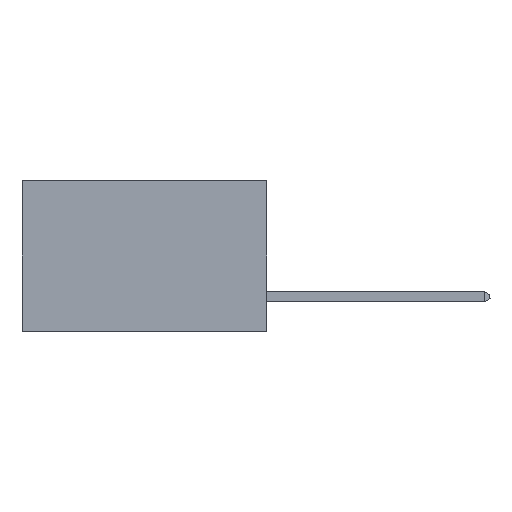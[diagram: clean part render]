
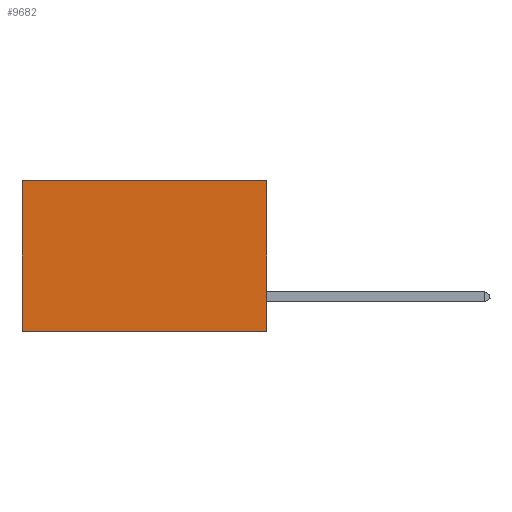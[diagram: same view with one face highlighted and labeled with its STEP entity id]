
A CAD part, left-side view. The second image highlights one B-rep face of the part: STEP entity #9682.
In plain terms, the highlighted planar face has unit normal (-1, 0, 0).
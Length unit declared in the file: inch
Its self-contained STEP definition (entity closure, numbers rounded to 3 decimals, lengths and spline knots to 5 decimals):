
#956 = CARTESIAN_POINT ( 'NONE',  ( 0.2875, 0., -0.37 ) ) ;
#1392 = EDGE_CURVE ( 'NONE', #4689, #6636, #9210, .T. ) ;
#2105 = CARTESIAN_POINT ( 'NONE',  ( 0.2875, 0., 0. ) ) ;
#2436 = CARTESIAN_POINT ( 'NONE',  ( 0.2875, 0.6, 0. ) ) ;
#4689 = VERTEX_POINT ( 'NONE', #9300 ) ;
#6636 = VERTEX_POINT ( 'NONE', #956 ) ;
#9111 = ORIENTED_EDGE ( 'NONE', *, *, #23193, .T. ) ;
#9210 = LINE ( 'NONE', #2105, #10890 ) ;
#9248 = CARTESIAN_POINT ( 'NONE',  ( 0.2875, 0.6, -0.37 ) ) ;
#9300 = CARTESIAN_POINT ( 'NONE',  ( 0.2875, 0., 0. ) ) ;
#9354 = LINE ( 'NONE', #16980, #9716 ) ;
#9682 = ADVANCED_FACE ( 'NONE', ( #26703 ), #21024, .F. ) ;
#9716 = VECTOR ( 'NONE', #25395, 39.37008 ) ;
#10189 = DIRECTION ( 'NONE',  ( 0., 0., -1. ) ) ;
#10890 = VECTOR ( 'NONE', #22115, 39.37008 ) ;
#11216 = DIRECTION ( 'NONE',  ( 0., 0., -1. ) ) ;
#11293 = LINE ( 'NONE', #2436, #22869 ) ;
#15219 = EDGE_CURVE ( 'NONE', #6636, #17281, #9354, .T. ) ;
#16893 = CARTESIAN_POINT ( 'NONE',  ( 0.2875, 0., 0. ) ) ;
#16980 = CARTESIAN_POINT ( 'NONE',  ( 0.2875, 0., -0.37 ) ) ;
#17281 = VERTEX_POINT ( 'NONE', #9248 ) ;
#17890 = EDGE_LOOP ( 'NONE', ( #9111, #19348, #21341, #23915 ) ) ;
#18639 = LINE ( 'NONE', #23963, #24464 ) ;
#18724 = DIRECTION ( 'NONE',  ( 1., 0., 0. ) ) ;
#19348 = ORIENTED_EDGE ( 'NONE', *, *, #15219, .F. ) ;
#21024 = PLANE ( 'NONE',  #23832 ) ;
#21341 = ORIENTED_EDGE ( 'NONE', *, *, #1392, .F. ) ;
#21384 = EDGE_CURVE ( 'NONE', #4689, #22201, #18639, .T. ) ;
#22115 = DIRECTION ( 'NONE',  ( 0., 0., -1. ) ) ;
#22201 = VERTEX_POINT ( 'NONE', #22796 ) ;
#22796 = CARTESIAN_POINT ( 'NONE',  ( 0.2875, 0.6, 0. ) ) ;
#22869 = VECTOR ( 'NONE', #11216, 39.37008 ) ;
#23193 = EDGE_CURVE ( 'NONE', #22201, #17281, #11293, .T. ) ;
#23832 = AXIS2_PLACEMENT_3D ( 'NONE', #16893, #18724, #10189 ) ;
#23915 = ORIENTED_EDGE ( 'NONE', *, *, #21384, .T. ) ;
#23963 = CARTESIAN_POINT ( 'NONE',  ( 0.2875, 0., 0. ) ) ;
#24464 = VECTOR ( 'NONE', #26182, 39.37008 ) ;
#25395 = DIRECTION ( 'NONE',  ( 0., 1., 0. ) ) ;
#26182 = DIRECTION ( 'NONE',  ( 0., 1., 0. ) ) ;
#26703 = FACE_OUTER_BOUND ( 'NONE', #17890, .T. ) ;
